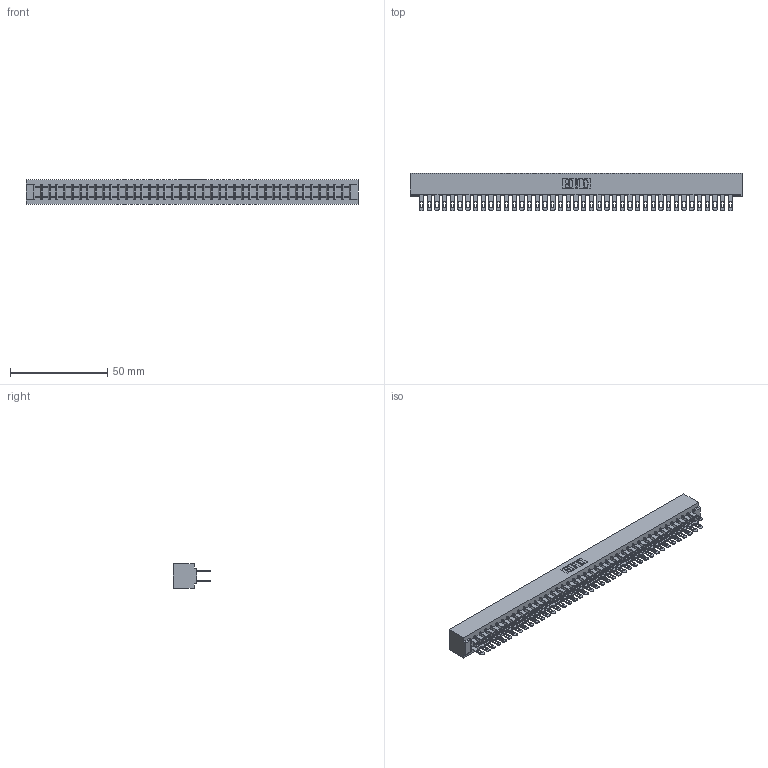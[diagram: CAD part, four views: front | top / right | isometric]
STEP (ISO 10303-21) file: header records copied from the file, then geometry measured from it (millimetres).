
FILE_DESCRIPTION (( 'STEP AP203' ), '1' );
FILE_NAME ('307-082-500-201.STEP', '2019-09-07T00:23:51', ( '' ), ( '' ), 'SwSTEP 2.0', 'SolidWorks 2016', '' );
FILE_SCHEMA (( 'CONFIG_CONTROL_DESIGN' ));
Length unit declared in the file: inch
Products named in the file (3): 307-290-001_500; 307-082-500-201; 307 Part_No Mounting Lugs
Assembly tree (83 placements, depth 2):
  307-082-500-201
    307 Part_No Mounting Lugs
    307-290-001_500  x82
Bounding box: 170.33 x 19.18 x 12.7 mm (x, y, z)
Volume: 18888.3 mm3; surface area: 24710.6 mm2
Topology: 83 solids, 83 shells, 3924 faces, 10959 edges, 7082 vertices
Faces by surface type: plane 2526, cylinder 1314, sphere 84
Entity records: 36280 total; most frequent: CARTESIAN_POINT 5929, ORIENTED_EDGE 5874, DIRECTION 5809, EDGE_CURVE 2937, LINE 2253, VECTOR 2253, VERTEX_POINT 1898, AXIS2_PLACEMENT_3D 1778
